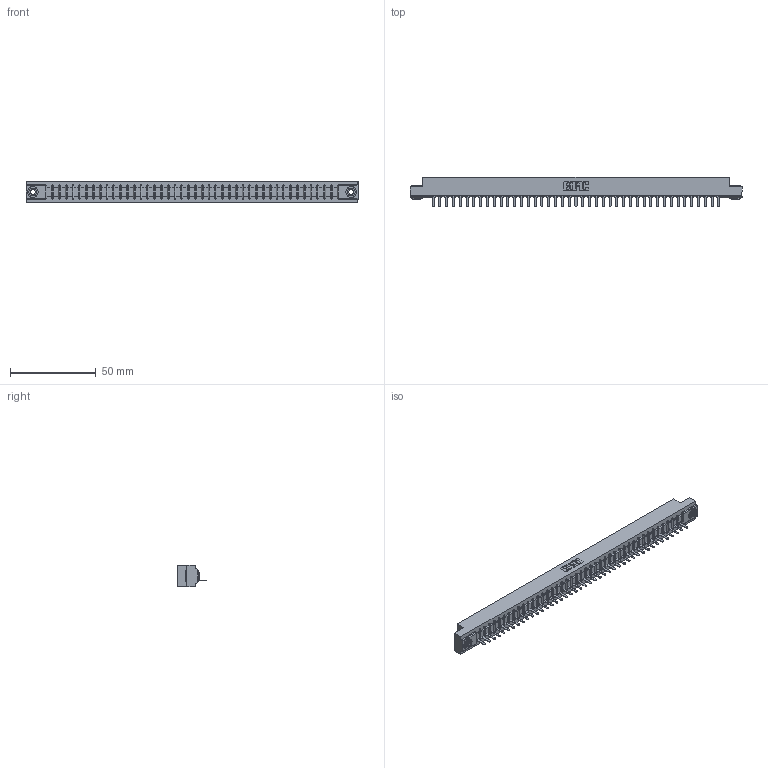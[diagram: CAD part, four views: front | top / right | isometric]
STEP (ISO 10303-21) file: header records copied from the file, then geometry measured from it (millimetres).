
FILE_DESCRIPTION (( 'STEP AP203' ), '1' );
FILE_NAME ('357-043-521-103.STEP', '2019-09-17T10:53:45', ( '' ), ( '' ), 'SwSTEP 2.0', 'SolidWorks 2016', '' );
FILE_SCHEMA (( 'CONFIG_CONTROL_DESIGN' ));
Length unit declared in the file: inch
Products named in the file (4): 307 Part_.156 Dia Mounting Holes; 345-250-002_345-250-002-102; 357-043-521-103; 307-290-002_521
Assembly tree (46 placements, depth 2):
  357-043-521-103
    307 Part_.156 Dia Mounting Holes
    307-290-002_521  x43
    345-250-002_345-250-002-102  x2
Bounding box: 193.4 x 17.42 x 12.7 mm (x, y, z)
Volume: 20707.1 mm3; surface area: 26314.4 mm2
Topology: 46 solids, 46 shells, 3396 faces, 10411 edges, 6818 vertices
Faces by surface type: plane 2029, cylinder 1271, sphere 88, cone 8
Entity records: 38523 total; most frequent: CARTESIAN_POINT 6477, ORIENTED_EDGE 6458, DIRECTION 6307, EDGE_CURVE 3229, VECTOR 2467, LINE 2467, VERTEX_POINT 2090, AXIS2_PLACEMENT_3D 1920
